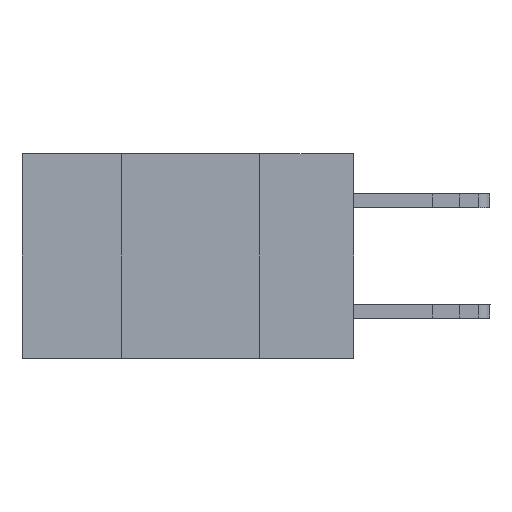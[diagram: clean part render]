
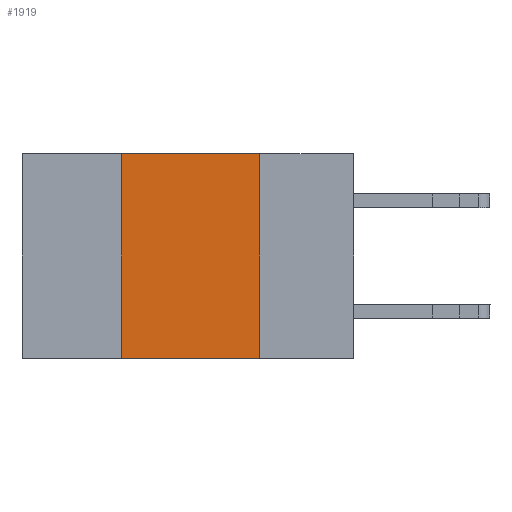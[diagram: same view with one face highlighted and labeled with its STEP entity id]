
A CAD part, left-side view. The second image highlights one B-rep face of the part: STEP entity #1919.
In plain terms, the highlighted planar face has unit normal (-1, 0, 0).
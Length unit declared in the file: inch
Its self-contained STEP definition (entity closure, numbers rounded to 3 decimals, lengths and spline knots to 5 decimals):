
#457 = ORIENTED_EDGE ( 'NONE', *, *, #18248, .F. ) ;
#752 = DIRECTION ( 'NONE',  ( 0., 0., -1. ) ) ;
#1919 = ADVANCED_FACE ( 'NONE', ( #15007 ), #4268, .F. ) ;
#3430 = AXIS2_PLACEMENT_3D ( 'NONE', #18609, #16743, #752 ) ;
#4268 = PLANE ( 'NONE',  #3430 ) ;
#4358 = CARTESIAN_POINT ( 'NONE',  ( 0., 0.17, 0. ) ) ;
#4561 = DIRECTION ( 'NONE',  ( 0., 0., -1. ) ) ;
#4968 = CARTESIAN_POINT ( 'NONE',  ( 0., 0.6, 0. ) ) ;
#6206 = VERTEX_POINT ( 'NONE', #14029 ) ;
#8278 = ORIENTED_EDGE ( 'NONE', *, *, #15949, .F. ) ;
#8665 = CARTESIAN_POINT ( 'NONE',  ( 0., 0.42, 0. ) ) ;
#9198 = LINE ( 'NONE', #8665, #23541 ) ;
#9742 = CARTESIAN_POINT ( 'NONE',  ( 0., 0.6, -0.37 ) ) ;
#11133 = VERTEX_POINT ( 'NONE', #18982 ) ;
#12608 = CARTESIAN_POINT ( 'NONE',  ( 0., 0.17, 0. ) ) ;
#14029 = CARTESIAN_POINT ( 'NONE',  ( 0., 0.42, 0. ) ) ;
#15007 = FACE_OUTER_BOUND ( 'NONE', #18973, .T. ) ;
#15287 = DIRECTION ( 'NONE',  ( 0., -1., 0. ) ) ;
#15777 = EDGE_CURVE ( 'NONE', #16841, #11133, #24953, .T. ) ;
#15949 = EDGE_CURVE ( 'NONE', #6206, #16841, #23202, .T. ) ;
#16047 = LINE ( 'NONE', #9742, #16338 ) ;
#16338 = VECTOR ( 'NONE', #24212, 39.37008 ) ;
#16743 = DIRECTION ( 'NONE',  ( 1., 0., 0. ) ) ;
#16841 = VERTEX_POINT ( 'NONE', #4358 ) ;
#17096 = DIRECTION ( 'NONE',  ( 0., 0., 1. ) ) ;
#18248 = EDGE_CURVE ( 'NONE', #19488, #6206, #9198, .T. ) ;
#18603 = ORIENTED_EDGE ( 'NONE', *, *, #26529, .T. ) ;
#18609 = CARTESIAN_POINT ( 'NONE',  ( 0., 0.6, 0. ) ) ;
#18973 = EDGE_LOOP ( 'NONE', ( #19736, #8278, #457, #18603 ) ) ;
#18982 = CARTESIAN_POINT ( 'NONE',  ( 0., 0.17, -0.37 ) ) ;
#19488 = VERTEX_POINT ( 'NONE', #23055 ) ;
#19736 = ORIENTED_EDGE ( 'NONE', *, *, #15777, .F. ) ;
#20102 = VECTOR ( 'NONE', #15287, 39.37008 ) ;
#23055 = CARTESIAN_POINT ( 'NONE',  ( 0., 0.42, -0.37 ) ) ;
#23108 = VECTOR ( 'NONE', #4561, 39.37008 ) ;
#23202 = LINE ( 'NONE', #4968, #20102 ) ;
#23541 = VECTOR ( 'NONE', #17096, 39.37008 ) ;
#24212 = DIRECTION ( 'NONE',  ( 0., -1., 0. ) ) ;
#24953 = LINE ( 'NONE', #12608, #23108 ) ;
#26529 = EDGE_CURVE ( 'NONE', #19488, #11133, #16047, .T. ) ;
